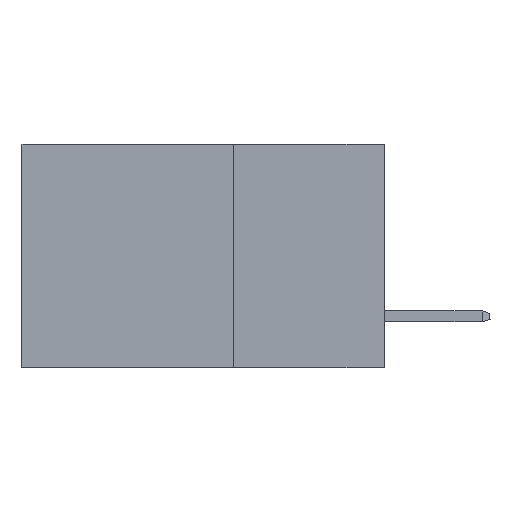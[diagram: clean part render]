
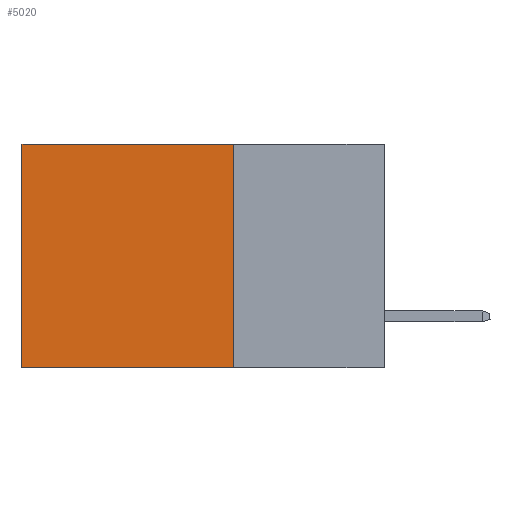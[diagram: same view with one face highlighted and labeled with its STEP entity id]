
A CAD part, left-side view. The second image highlights one B-rep face of the part: STEP entity #5020.
In plain terms, the highlighted planar face has unit normal (-1, 0, 0).
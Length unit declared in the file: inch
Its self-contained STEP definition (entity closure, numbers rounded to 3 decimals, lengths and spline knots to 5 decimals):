
#1291 = CARTESIAN_POINT ( 'NONE',  ( 0.298, 0.25, -0.37 ) ) ;
#1543 = DIRECTION ( 'NONE',  ( 1., 0., 0. ) ) ;
#2083 = LINE ( 'NONE', #1291, #7626 ) ;
#2975 = VERTEX_POINT ( 'NONE', #15027 ) ;
#3489 = AXIS2_PLACEMENT_3D ( 'NONE', #25156, #1543, #18150 ) ;
#3721 = DIRECTION ( 'NONE',  ( 0., 1., 0. ) ) ;
#5020 = ADVANCED_FACE ( 'NONE', ( #10834 ), #15752, .F. ) ;
#5181 = ORIENTED_EDGE ( 'NONE', *, *, #12011, .F. ) ;
#5880 = VERTEX_POINT ( 'NONE', #11788 ) ;
#6124 = CARTESIAN_POINT ( 'NONE',  ( 0.298, 0.6, -0.37 ) ) ;
#6314 = CARTESIAN_POINT ( 'NONE',  ( 0.298, 0.25, 0. ) ) ;
#7626 = VECTOR ( 'NONE', #3721, 39.37008 ) ;
#9053 = VERTEX_POINT ( 'NONE', #12810 ) ;
#9120 = EDGE_CURVE ( 'NONE', #5880, #22547, #2083, .T. ) ;
#10834 = FACE_OUTER_BOUND ( 'NONE', #16996, .T. ) ;
#10910 = DIRECTION ( 'NONE',  ( 0., 0., -1. ) ) ;
#11702 = ORIENTED_EDGE ( 'NONE', *, *, #16183, .T. ) ;
#11788 = CARTESIAN_POINT ( 'NONE',  ( 0.298, 0.25, -0.37 ) ) ;
#12011 = EDGE_CURVE ( 'NONE', #9053, #5880, #26900, .T. ) ;
#12237 = ORIENTED_EDGE ( 'NONE', *, *, #9120, .F. ) ;
#12810 = CARTESIAN_POINT ( 'NONE',  ( 0.298, 0.25, 0. ) ) ;
#13106 = DIRECTION ( 'NONE',  ( 0., 0., -1. ) ) ;
#14761 = VECTOR ( 'NONE', #10910, 39.37008 ) ;
#15027 = CARTESIAN_POINT ( 'NONE',  ( 0.298, 0.6, 0. ) ) ;
#15391 = CARTESIAN_POINT ( 'NONE',  ( 0.298, 0.25, 0. ) ) ;
#15744 = DIRECTION ( 'NONE',  ( 0., 1., 0. ) ) ;
#15752 = PLANE ( 'NONE',  #3489 ) ;
#16183 = EDGE_CURVE ( 'NONE', #9053, #2975, #18263, .T. ) ;
#16996 = EDGE_LOOP ( 'NONE', ( #17617, #12237, #5181, #11702 ) ) ;
#17617 = ORIENTED_EDGE ( 'NONE', *, *, #18599, .T. ) ;
#18150 = DIRECTION ( 'NONE',  ( 0., 0., -1. ) ) ;
#18263 = LINE ( 'NONE', #6314, #23805 ) ;
#18599 = EDGE_CURVE ( 'NONE', #2975, #22547, #26549, .T. ) ;
#20466 = CARTESIAN_POINT ( 'NONE',  ( 0.298, 0.6, 0. ) ) ;
#22547 = VERTEX_POINT ( 'NONE', #6124 ) ;
#23805 = VECTOR ( 'NONE', #15744, 39.37008 ) ;
#25156 = CARTESIAN_POINT ( 'NONE',  ( 0.298, 0.25, 0. ) ) ;
#25451 = VECTOR ( 'NONE', #13106, 39.37008 ) ;
#26549 = LINE ( 'NONE', #20466, #14761 ) ;
#26900 = LINE ( 'NONE', #15391, #25451 ) ;
